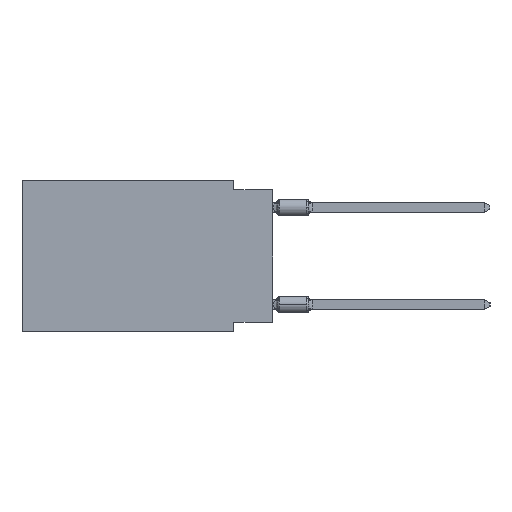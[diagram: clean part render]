
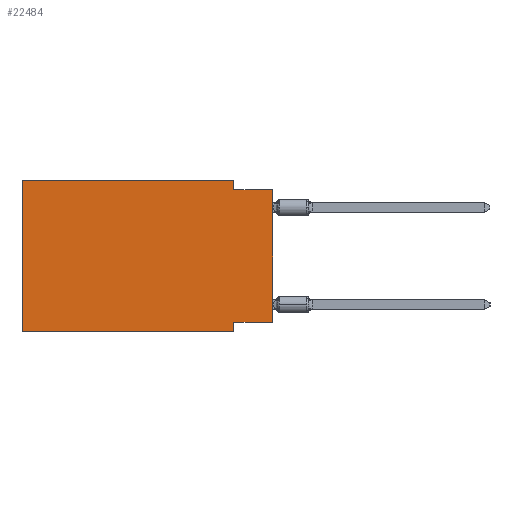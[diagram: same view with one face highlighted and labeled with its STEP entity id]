
A CAD part, left-side view. The second image highlights one B-rep face of the part: STEP entity #22484.
In plain terms, the highlighted planar face has unit normal (-1, 0, 0).
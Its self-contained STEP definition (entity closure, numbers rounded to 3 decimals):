
#838 = VECTOR ( 'NONE', #44764, 1000. ) ;
#1497 = CARTESIAN_POINT ( 'NONE',  ( 0., 16.383, 0. ) ) ;
#1740 = DIRECTION ( 'NONE',  ( 0., -1., 0. ) ) ;
#1895 = VERTEX_POINT ( 'NONE', #36793 ) ;
#2203 = DIRECTION ( 'NONE',  ( 1., 0., 0. ) ) ;
#2448 = FACE_OUTER_BOUND ( 'NONE', #22309, .T. ) ;
#3280 = LINE ( 'NONE', #43077, #19193 ) ;
#5535 = VERTEX_POINT ( 'NONE', #10045 ) ;
#5724 = EDGE_CURVE ( 'NONE', #50620, #6432, #28239, .T. ) ;
#6003 = CARTESIAN_POINT ( 'NONE',  ( 0., 0., -0.635 ) ) ;
#6184 = VECTOR ( 'NONE', #12998, 1000. ) ;
#6432 = VERTEX_POINT ( 'NONE', #46644 ) ;
#6624 = ORIENTED_EDGE ( 'NONE', *, *, #40286, .F. ) ;
#7071 = VECTOR ( 'NONE', #1740, 1000. ) ;
#8354 = CARTESIAN_POINT ( 'NONE',  ( 0., 2.54, -9.271 ) ) ;
#8731 = EDGE_CURVE ( 'NONE', #34457, #37667, #25445, .T. ) ;
#10045 = CARTESIAN_POINT ( 'NONE',  ( 0., 2.54, -9.906 ) ) ;
#10781 = CARTESIAN_POINT ( 'NONE',  ( 0., 0., -0.635 ) ) ;
#12113 = LINE ( 'NONE', #27772, #32271 ) ;
#12465 = VECTOR ( 'NONE', #14986, 1000. ) ;
#12998 = DIRECTION ( 'NONE',  ( 0., 0., -1. ) ) ;
#13500 = DIRECTION ( 'NONE',  ( 0., 0., -1. ) ) ;
#14683 = ORIENTED_EDGE ( 'NONE', *, *, #35042, .F. ) ;
#14986 = DIRECTION ( 'NONE',  ( 0., 0., 1. ) ) ;
#16407 = VECTOR ( 'NONE', #30318, 1000. ) ;
#16512 = VECTOR ( 'NONE', #45396, 1000. ) ;
#16914 = EDGE_CURVE ( 'NONE', #34457, #34875, #37456, .T. ) ;
#18395 = VERTEX_POINT ( 'NONE', #21205 ) ;
#19193 = VECTOR ( 'NONE', #46448, 1000. ) ;
#21205 = CARTESIAN_POINT ( 'NONE',  ( 0., 2.54, -0.635 ) ) ;
#22012 = EDGE_CURVE ( 'NONE', #37667, #5535, #12113, .T. ) ;
#22309 = EDGE_LOOP ( 'NONE', ( #41462, #40328, #6624, #25717, #14683, #32407, #40324, #28615 ) ) ;
#22484 = ADVANCED_FACE ( 'NONE', ( #2448 ), #28908, .F. ) ;
#23798 = LINE ( 'NONE', #35609, #6184 ) ;
#25445 = LINE ( 'NONE', #44969, #16407 ) ;
#25717 = ORIENTED_EDGE ( 'NONE', *, *, #5724, .F. ) ;
#26049 = CARTESIAN_POINT ( 'NONE',  ( 0., 16.383, 0. ) ) ;
#27772 = CARTESIAN_POINT ( 'NONE',  ( 0., 2.54, -9.906 ) ) ;
#28239 = LINE ( 'NONE', #1497, #7071 ) ;
#28615 = ORIENTED_EDGE ( 'NONE', *, *, #8731, .F. ) ;
#28908 = PLANE ( 'NONE',  #33898 ) ;
#30318 = DIRECTION ( 'NONE',  ( 0., 1., 0. ) ) ;
#32271 = VECTOR ( 'NONE', #39596, 1000. ) ;
#32407 = ORIENTED_EDGE ( 'NONE', *, *, #43244, .T. ) ;
#32734 = EDGE_CURVE ( 'NONE', #18395, #34875, #45985, .T. ) ;
#33284 = CARTESIAN_POINT ( 'NONE',  ( 0., 16.383, 0. ) ) ;
#33898 = AXIS2_PLACEMENT_3D ( 'NONE', #33284, #2203, #13500 ) ;
#34457 = VERTEX_POINT ( 'NONE', #43343 ) ;
#34875 = VERTEX_POINT ( 'NONE', #6003 ) ;
#35042 = EDGE_CURVE ( 'NONE', #1895, #50620, #38622, .T. ) ;
#35609 = CARTESIAN_POINT ( 'NONE',  ( 0., 2.54, 0. ) ) ;
#36793 = CARTESIAN_POINT ( 'NONE',  ( 0., 16.383, -9.906 ) ) ;
#37456 = LINE ( 'NONE', #49780, #16512 ) ;
#37667 = VERTEX_POINT ( 'NONE', #8354 ) ;
#38622 = LINE ( 'NONE', #26049, #12465 ) ;
#39596 = DIRECTION ( 'NONE',  ( 0., 0., -1. ) ) ;
#40286 = EDGE_CURVE ( 'NONE', #6432, #18395, #23798, .T. ) ;
#40324 = ORIENTED_EDGE ( 'NONE', *, *, #22012, .F. ) ;
#40328 = ORIENTED_EDGE ( 'NONE', *, *, #32734, .F. ) ;
#41462 = ORIENTED_EDGE ( 'NONE', *, *, #16914, .T. ) ;
#43077 = CARTESIAN_POINT ( 'NONE',  ( 0., 16.383, -9.906 ) ) ;
#43244 = EDGE_CURVE ( 'NONE', #1895, #5535, #3280, .T. ) ;
#43343 = CARTESIAN_POINT ( 'NONE',  ( 0., 0., -9.271 ) ) ;
#44764 = DIRECTION ( 'NONE',  ( 0., -1., 0. ) ) ;
#44969 = CARTESIAN_POINT ( 'NONE',  ( 0., 0., -9.271 ) ) ;
#45396 = DIRECTION ( 'NONE',  ( 0., 0., 1. ) ) ;
#45985 = LINE ( 'NONE', #10781, #838 ) ;
#46448 = DIRECTION ( 'NONE',  ( 0., -1., 0. ) ) ;
#46644 = CARTESIAN_POINT ( 'NONE',  ( 0., 2.54, 0. ) ) ;
#47740 = CARTESIAN_POINT ( 'NONE',  ( 0., 16.383, 0. ) ) ;
#49780 = CARTESIAN_POINT ( 'NONE',  ( 0., 0., 0. ) ) ;
#50620 = VERTEX_POINT ( 'NONE', #47740 ) ;
